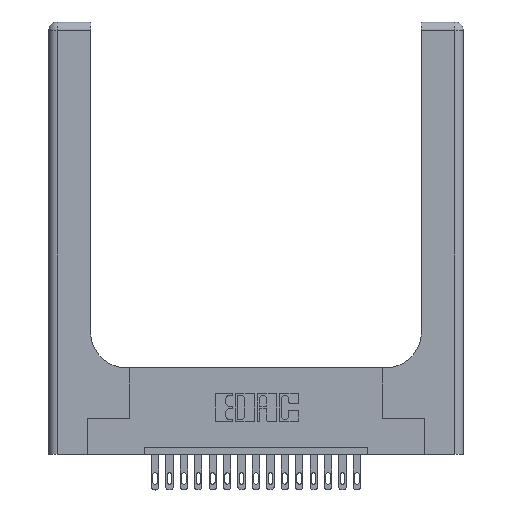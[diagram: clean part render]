
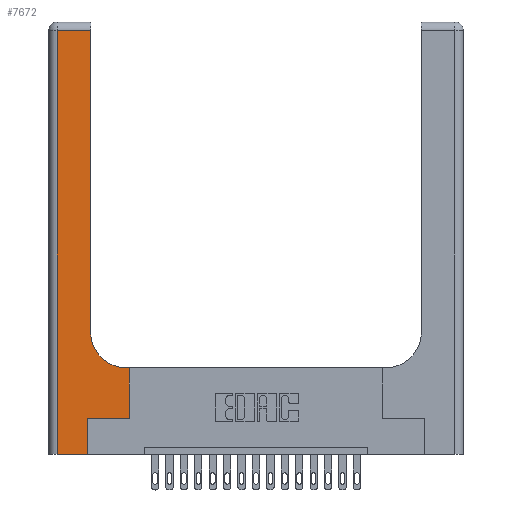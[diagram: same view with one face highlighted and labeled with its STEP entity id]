
A CAD part, top view. The second image highlights one B-rep face of the part: STEP entity #7672.
In plain terms, the highlighted planar face has unit normal (0, 0, 1).
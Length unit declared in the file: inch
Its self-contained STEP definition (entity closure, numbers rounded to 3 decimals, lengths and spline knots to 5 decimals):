
#307 = DIRECTION ( 'NONE',  ( 1., 0., 0. ) ) ;
#468 = VECTOR ( 'NONE', #307, 39.37008 ) ;
#852 = CARTESIAN_POINT ( 'NONE',  ( 0.2915, 0.6, 0.37 ) ) ;
#1367 = VECTOR ( 'NONE', #17983, 39.37008 ) ;
#1939 = VERTEX_POINT ( 'NONE', #18030 ) ;
#3240 = DIRECTION ( 'NONE',  ( 0., 1., 0. ) ) ;
#3264 = DIRECTION ( 'NONE',  ( 0., 0., -1. ) ) ;
#3309 = DIRECTION ( 'NONE',  ( 0., 0., -1. ) ) ;
#3497 = VERTEX_POINT ( 'NONE', #19611 ) ;
#3525 = CARTESIAN_POINT ( 'NONE',  ( 0.5585, 0.25, 0.37 ) ) ;
#3613 = LINE ( 'NONE', #13729, #16622 ) ;
#3659 = DIRECTION ( 'NONE',  ( 0., 1., 0. ) ) ;
#3672 = VECTOR ( 'NONE', #10514, 39.37008 ) ;
#4019 = ORIENTED_EDGE ( 'NONE', *, *, #8812, .T. ) ;
#4370 = LINE ( 'NONE', #13855, #8699 ) ;
#4495 = LINE ( 'NONE', #852, #1367 ) ;
#4609 = DIRECTION ( 'NONE',  ( 0., -1., 0. ) ) ;
#4726 = DIRECTION ( 'NONE',  ( -1., 0., 0. ) ) ;
#4806 = DIRECTION ( 'NONE',  ( 1., 0., 0. ) ) ;
#5627 = ORIENTED_EDGE ( 'NONE', *, *, #13012, .T. ) ;
#5844 = VERTEX_POINT ( 'NONE', #16429 ) ;
#6339 = EDGE_CURVE ( 'NONE', #3497, #5844, #4495, .T. ) ;
#6420 = ORIENTED_EDGE ( 'NONE', *, *, #10948, .T. ) ;
#6604 = AXIS2_PLACEMENT_3D ( 'NONE', #10864, #3309, #4726 ) ;
#7341 = AXIS2_PLACEMENT_3D ( 'NONE', #12489, #3264, #4806 ) ;
#7637 = CARTESIAN_POINT ( 'NONE',  ( 0.2915, 3., 0.37 ) ) ;
#7672 = ADVANCED_FACE ( 'NONE', ( #18200 ), #13957, .F. ) ;
#7839 = VECTOR ( 'NONE', #3240, 39.37008 ) ;
#8699 = VECTOR ( 'NONE', #4609, 39.37008 ) ;
#8812 = EDGE_CURVE ( 'NONE', #11091, #3497, #18325, .T. ) ;
#9139 = LINE ( 'NONE', #9603, #468 ) ;
#9603 = CARTESIAN_POINT ( 'NONE',  ( 0.269, 0.25, 0.37 ) ) ;
#10003 = CARTESIAN_POINT ( 'NONE',  ( 0.2915, 0.85, 0.37 ) ) ;
#10355 = DIRECTION ( 'NONE',  ( 1., 0., 0. ) ) ;
#10514 = DIRECTION ( 'NONE',  ( -1., 0., 0. ) ) ;
#10784 = ORIENTED_EDGE ( 'NONE', *, *, #15919, .T. ) ;
#10864 = CARTESIAN_POINT ( 'NONE',  ( 0., 3., 0.37 ) ) ;
#10948 = EDGE_CURVE ( 'NONE', #18774, #1939, #17893, .T. ) ;
#11091 = VERTEX_POINT ( 'NONE', #3525 ) ;
#11279 = CARTESIAN_POINT ( 'NONE',  ( 0.5585, 0.25, 0.37 ) ) ;
#11595 = ORIENTED_EDGE ( 'NONE', *, *, #15278, .T. ) ;
#12489 = CARTESIAN_POINT ( 'NONE',  ( 0.5415, 0.85, 0.37 ) ) ;
#12896 = CARTESIAN_POINT ( 'NONE',  ( 0.06, 2.94, 0.37 ) ) ;
#13012 = EDGE_CURVE ( 'NONE', #1939, #17429, #16430, .T. ) ;
#13463 = CIRCLE ( 'NONE', #7341, 0.25 ) ;
#13576 = ORIENTED_EDGE ( 'NONE', *, *, #14048, .T. ) ;
#13729 = CARTESIAN_POINT ( 'NONE',  ( 0., 0., 0.37 ) ) ;
#13844 = DIRECTION ( 'NONE',  ( 0., 1., 0. ) ) ;
#13855 = CARTESIAN_POINT ( 'NONE',  ( 0.06, 3., 0.37 ) ) ;
#13928 = ORIENTED_EDGE ( 'NONE', *, *, #14745, .T. ) ;
#13957 = PLANE ( 'NONE',  #6604 ) ;
#14015 = VECTOR ( 'NONE', #13844, 39.37008 ) ;
#14048 = EDGE_CURVE ( 'NONE', #17429, #15981, #4370, .T. ) ;
#14216 = VECTOR ( 'NONE', #3659, 39.37008 ) ;
#14301 = CARTESIAN_POINT ( 'NONE',  ( 0.269, 0., 0.37 ) ) ;
#14623 = LINE ( 'NONE', #14301, #7839 ) ;
#14726 = ORIENTED_EDGE ( 'NONE', *, *, #15088, .T. ) ;
#14745 = EDGE_CURVE ( 'NONE', #17243, #16832, #14623, .T. ) ;
#15088 = EDGE_CURVE ( 'NONE', #15981, #17243, #3613, .T. ) ;
#15092 = CARTESIAN_POINT ( 'NONE',  ( 0., 2.94, 0.37 ) ) ;
#15244 = ORIENTED_EDGE ( 'NONE', *, *, #6339, .T. ) ;
#15278 = EDGE_CURVE ( 'NONE', #16832, #11091, #9139, .T. ) ;
#15919 = EDGE_CURVE ( 'NONE', #5844, #18774, #13463, .T. ) ;
#15981 = VERTEX_POINT ( 'NONE', #19066 ) ;
#16429 = CARTESIAN_POINT ( 'NONE',  ( 0.5415, 0.6, 0.37 ) ) ;
#16430 = LINE ( 'NONE', #15092, #3672 ) ;
#16622 = VECTOR ( 'NONE', #10355, 39.37008 ) ;
#16832 = VERTEX_POINT ( 'NONE', #17829 ) ;
#17010 = EDGE_LOOP ( 'NONE', ( #6420, #5627, #13576, #14726, #13928, #11595, #4019, #15244, #10784 ) ) ;
#17243 = VERTEX_POINT ( 'NONE', #18649 ) ;
#17429 = VERTEX_POINT ( 'NONE', #12896 ) ;
#17829 = CARTESIAN_POINT ( 'NONE',  ( 0.269, 0.25, 0.37 ) ) ;
#17893 = LINE ( 'NONE', #7637, #14015 ) ;
#17983 = DIRECTION ( 'NONE',  ( -1., 0., 0. ) ) ;
#18030 = CARTESIAN_POINT ( 'NONE',  ( 0.2915, 2.94, 0.37 ) ) ;
#18200 = FACE_OUTER_BOUND ( 'NONE', #17010, .T. ) ;
#18325 = LINE ( 'NONE', #11279, #14216 ) ;
#18649 = CARTESIAN_POINT ( 'NONE',  ( 0.269, 0., 0.37 ) ) ;
#18774 = VERTEX_POINT ( 'NONE', #10003 ) ;
#19066 = CARTESIAN_POINT ( 'NONE',  ( 0.06, 0., 0.37 ) ) ;
#19611 = CARTESIAN_POINT ( 'NONE',  ( 0.5585, 0.6, 0.37 ) ) ;
